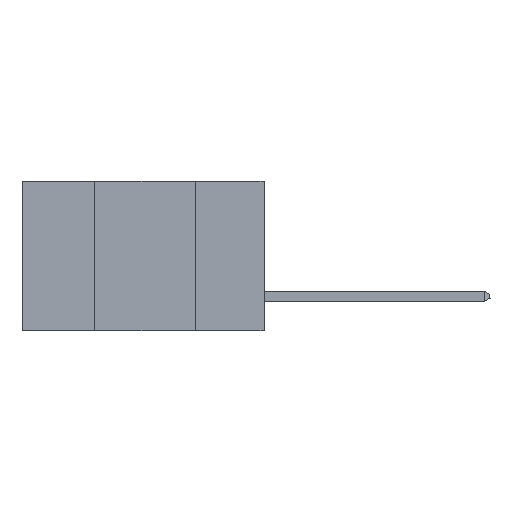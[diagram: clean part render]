
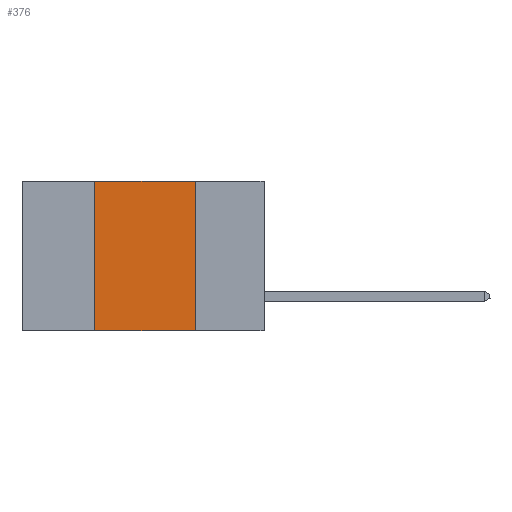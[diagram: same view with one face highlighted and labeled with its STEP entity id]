
A CAD part, left-side view. The second image highlights one B-rep face of the part: STEP entity #376.
In plain terms, the highlighted planar face has unit normal (-1, 0, 0).
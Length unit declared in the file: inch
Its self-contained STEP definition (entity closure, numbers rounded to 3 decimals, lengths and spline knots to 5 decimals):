
#327 = EDGE_CURVE ( 'NONE', #9820, #4583, #6158, .T. ) ;
#376 = ADVANCED_FACE ( 'NONE', ( #2765 ), #1660, .F. ) ;
#410 = DIRECTION ( 'NONE',  ( 0., -1., 0. ) ) ;
#550 = ORIENTED_EDGE ( 'NONE', *, *, #1482, .T. ) ;
#1482 = EDGE_CURVE ( 'NONE', #9820, #7243, #3285, .T. ) ;
#1660 = PLANE ( 'NONE',  #9320 ) ;
#1684 = EDGE_CURVE ( 'NONE', #4583, #9967, #11015, .T. ) ;
#1712 = ORIENTED_EDGE ( 'NONE', *, *, #1684, .F. ) ;
#1917 = CARTESIAN_POINT ( 'NONE',  ( 0., 0.17, 0. ) ) ;
#2165 = CARTESIAN_POINT ( 'NONE',  ( 0., 0.6, -0.37 ) ) ;
#2458 = VECTOR ( 'NONE', #5865, 39.37008 ) ;
#2593 = VECTOR ( 'NONE', #9368, 39.37008 ) ;
#2765 = FACE_OUTER_BOUND ( 'NONE', #7350, .T. ) ;
#3285 = LINE ( 'NONE', #2165, #5039 ) ;
#4133 = DIRECTION ( 'NONE',  ( 0., 0., 1. ) ) ;
#4583 = VERTEX_POINT ( 'NONE', #5874 ) ;
#5039 = VECTOR ( 'NONE', #410, 39.37008 ) ;
#5123 = ORIENTED_EDGE ( 'NONE', *, *, #7689, .F. ) ;
#5865 = DIRECTION ( 'NONE',  ( 0., -1., 0. ) ) ;
#5874 = CARTESIAN_POINT ( 'NONE',  ( 0., 0.42, 0. ) ) ;
#6158 = LINE ( 'NONE', #8569, #10388 ) ;
#6949 = DIRECTION ( 'NONE',  ( 0., 0., -1. ) ) ;
#7194 = LINE ( 'NONE', #8491, #2593 ) ;
#7243 = VERTEX_POINT ( 'NONE', #9000 ) ;
#7350 = EDGE_LOOP ( 'NONE', ( #5123, #1712, #9237, #550 ) ) ;
#7689 = EDGE_CURVE ( 'NONE', #9967, #7243, #7194, .T. ) ;
#7788 = DIRECTION ( 'NONE',  ( 1., 0., 0. ) ) ;
#8491 = CARTESIAN_POINT ( 'NONE',  ( 0., 0.17, 0. ) ) ;
#8537 = CARTESIAN_POINT ( 'NONE',  ( 0., 0.6, 0. ) ) ;
#8569 = CARTESIAN_POINT ( 'NONE',  ( 0., 0.42, 0. ) ) ;
#9000 = CARTESIAN_POINT ( 'NONE',  ( 0., 0.17, -0.37 ) ) ;
#9237 = ORIENTED_EDGE ( 'NONE', *, *, #327, .F. ) ;
#9320 = AXIS2_PLACEMENT_3D ( 'NONE', #8537, #7788, #6949 ) ;
#9368 = DIRECTION ( 'NONE',  ( 0., 0., -1. ) ) ;
#9820 = VERTEX_POINT ( 'NONE', #10199 ) ;
#9967 = VERTEX_POINT ( 'NONE', #1917 ) ;
#10127 = CARTESIAN_POINT ( 'NONE',  ( 0., 0.6, 0. ) ) ;
#10199 = CARTESIAN_POINT ( 'NONE',  ( 0., 0.42, -0.37 ) ) ;
#10388 = VECTOR ( 'NONE', #4133, 39.37008 ) ;
#11015 = LINE ( 'NONE', #10127, #2458 ) ;
